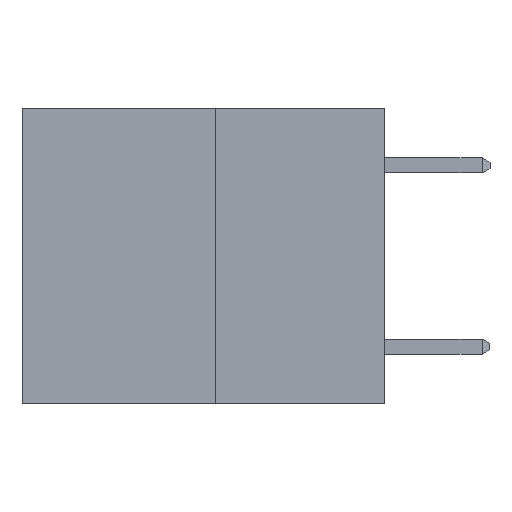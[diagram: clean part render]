
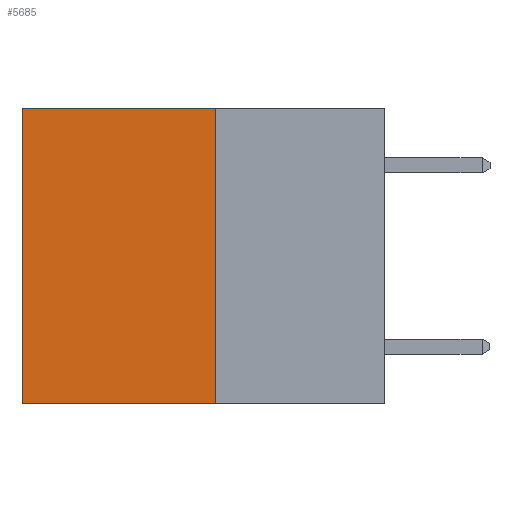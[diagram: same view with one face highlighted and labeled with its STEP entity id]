
A CAD part, left-side view. The second image highlights one B-rep face of the part: STEP entity #5685.
In plain terms, the highlighted planar face has unit normal (-1, 0, 0).
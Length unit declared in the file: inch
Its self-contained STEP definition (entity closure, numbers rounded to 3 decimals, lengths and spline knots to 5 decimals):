
#232 = FACE_OUTER_BOUND ( 'NONE', #9223, .T. ) ;
#517 = VERTEX_POINT ( 'NONE', #6395 ) ;
#636 = DIRECTION ( 'NONE',  ( 1., 0., 0. ) ) ;
#1298 = ORIENTED_EDGE ( 'NONE', *, *, #5613, .F. ) ;
#2057 = VECTOR ( 'NONE', #9824, 39.37008 ) ;
#2654 = LINE ( 'NONE', #2680, #15171 ) ;
#2680 = CARTESIAN_POINT ( 'NONE',  ( 0.3165, 0.6, -0.49 ) ) ;
#3589 = DIRECTION ( 'NONE',  ( 0., 0., -1. ) ) ;
#3877 = ORIENTED_EDGE ( 'NONE', *, *, #8438, .T. ) ;
#4228 = LINE ( 'NONE', #12318, #2057 ) ;
#5489 = EDGE_CURVE ( 'NONE', #517, #5800, #2654, .T. ) ;
#5613 = EDGE_CURVE ( 'NONE', #13212, #7333, #4228, .T. ) ;
#5685 = ADVANCED_FACE ( 'NONE', ( #232 ), #13695, .F. ) ;
#5800 = VERTEX_POINT ( 'NONE', #15243 ) ;
#6395 = CARTESIAN_POINT ( 'NONE',  ( 0.3165, 0.6, 0. ) ) ;
#6565 = DIRECTION ( 'NONE',  ( 0., 0., -1. ) ) ;
#6889 = CARTESIAN_POINT ( 'NONE',  ( 0.3165, 0.28, 0. ) ) ;
#7333 = VERTEX_POINT ( 'NONE', #12647 ) ;
#7668 = VECTOR ( 'NONE', #13785, 39.37008 ) ;
#7679 = ORIENTED_EDGE ( 'NONE', *, *, #13784, .F. ) ;
#8438 = EDGE_CURVE ( 'NONE', #13212, #517, #12762, .T. ) ;
#9223 = EDGE_LOOP ( 'NONE', ( #16231, #7679, #1298, #3877 ) ) ;
#9424 = DIRECTION ( 'NONE',  ( 0., 1., 0. ) ) ;
#9824 = DIRECTION ( 'NONE',  ( 0., 0., -1. ) ) ;
#9993 = CARTESIAN_POINT ( 'NONE',  ( 0.3165, 0.28, -0.49 ) ) ;
#11009 = LINE ( 'NONE', #9993, #7668 ) ;
#11100 = CARTESIAN_POINT ( 'NONE',  ( 0.3165, 0.28, -0.49 ) ) ;
#12288 = AXIS2_PLACEMENT_3D ( 'NONE', #11100, #636, #3589 ) ;
#12318 = CARTESIAN_POINT ( 'NONE',  ( 0.3165, 0.28, -0.49 ) ) ;
#12647 = CARTESIAN_POINT ( 'NONE',  ( 0.3165, 0.28, -0.49 ) ) ;
#12762 = LINE ( 'NONE', #6889, #13942 ) ;
#13212 = VERTEX_POINT ( 'NONE', #14469 ) ;
#13695 = PLANE ( 'NONE',  #12288 ) ;
#13784 = EDGE_CURVE ( 'NONE', #7333, #5800, #11009, .T. ) ;
#13785 = DIRECTION ( 'NONE',  ( 0., 1., 0. ) ) ;
#13942 = VECTOR ( 'NONE', #9424, 39.37008 ) ;
#14469 = CARTESIAN_POINT ( 'NONE',  ( 0.3165, 0.28, 0. ) ) ;
#15171 = VECTOR ( 'NONE', #6565, 39.37008 ) ;
#15243 = CARTESIAN_POINT ( 'NONE',  ( 0.3165, 0.6, -0.49 ) ) ;
#16231 = ORIENTED_EDGE ( 'NONE', *, *, #5489, .T. ) ;
